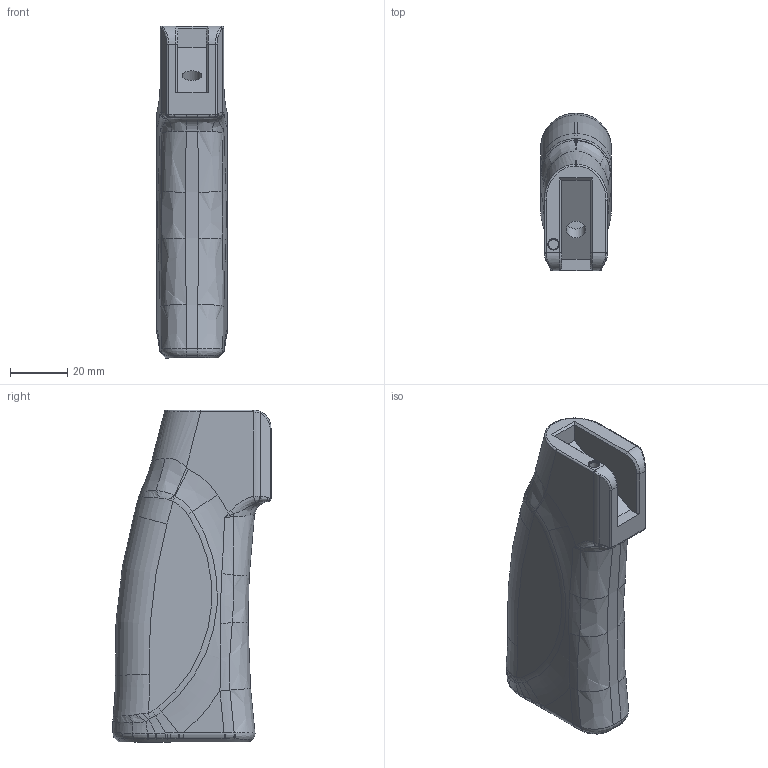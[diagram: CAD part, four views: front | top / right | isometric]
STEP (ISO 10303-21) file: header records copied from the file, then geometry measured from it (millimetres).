
FILE_DESCRIPTION(/* description */ (''),/* implementation_level */ '2;1');
FILE_NAME(/* name */ '3FTech 0 Degree Grip.step',/* time_stamp */ '2021-09-13T13:03:28-04:00',/* author */ (''),/* organization */ (''),/* preprocessor_version */ 'ST-DEVELOPER v18.1',/* originating_system */ 'Autodesk Translation Framework v10.10.0.1391',/* authorisation */ '');
FILE_SCHEMA (('AUTOMOTIVE_DESIGN { 1 0 10303 214 3 1 1 }'));
Length unit declared in the file: millimetre
Products named in the file (1): 3FTech 0 Degree Grip
Bounding box: 24.83 x 55.42 x 116.41 mm (x, y, z)
Volume: 55675.6 mm3; surface area: 26357.8 mm2
Topology: 1 solids, 1 shells, 379 faces, 921 edges, 546 vertices
Faces by surface type: bspline 233, torus 59, plane 45, cylinder 38, cone 4
Full cylindrical faces by diameter (mm): 3.4 x1, 6.8 x1, 15.489 x1
Entity records: 17882 total; most frequent: CARTESIAN_POINT 10314, ORIENTED_EDGE 1826, DIRECTION 1143, EDGE_CURVE 913, VERTEX_POINT 546, AXIS2_PLACEMENT_3D 494, B_SPLINE_CURVE_WITH_KNOTS 411, EDGE_LOOP 391
